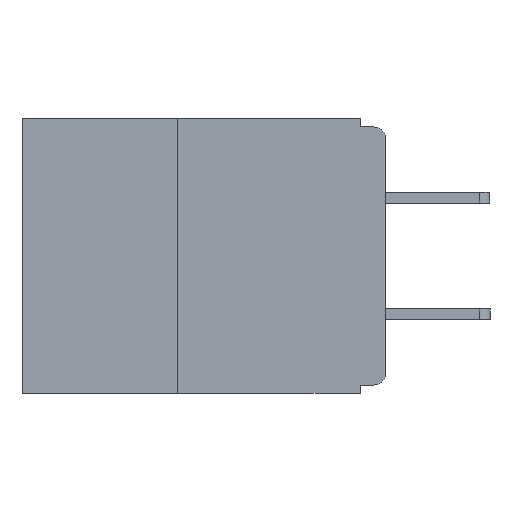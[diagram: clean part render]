
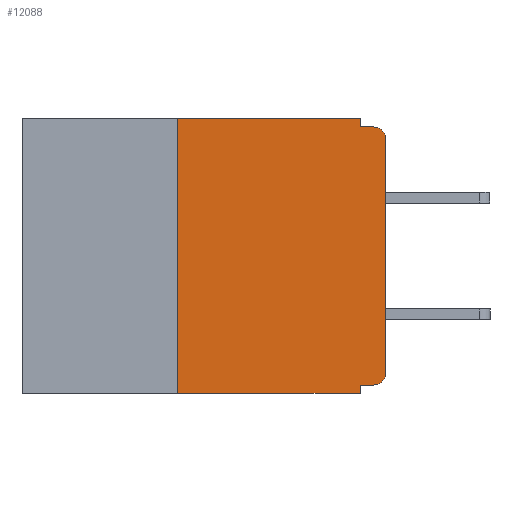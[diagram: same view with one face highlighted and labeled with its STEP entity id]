
A CAD part, left-side view. The second image highlights one B-rep face of the part: STEP entity #12088.
In plain terms, the highlighted planar face has unit normal (-1, 0, 0).
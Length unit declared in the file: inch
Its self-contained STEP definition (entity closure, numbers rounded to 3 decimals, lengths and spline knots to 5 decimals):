
#618 = VECTOR ( 'NONE', #12654, 39.37008 ) ;
#754 = DIRECTION ( 'NONE',  ( -1., 0., 0. ) ) ;
#861 = DIRECTION ( 'NONE',  ( 0., -1., 0. ) ) ;
#1012 = VECTOR ( 'NONE', #10283, 39.37008 ) ;
#1029 = EDGE_CURVE ( 'NONE', #26435, #22996, #21744, .T. ) ;
#1649 = ORIENTED_EDGE ( 'NONE', *, *, #1029, .T. ) ;
#1729 = LINE ( 'NONE', #7966, #1012 ) ;
#2002 = VECTOR ( 'NONE', #13486, 39.37008 ) ;
#2051 = EDGE_CURVE ( 'NONE', #28417, #3940, #6034, .T. ) ;
#2320 = LINE ( 'NONE', #24086, #21237 ) ;
#3777 = CARTESIAN_POINT ( 'NONE',  ( 0., 0.25, 0. ) ) ;
#3940 = VERTEX_POINT ( 'NONE', #28882 ) ;
#4041 = VECTOR ( 'NONE', #9494, 39.37008 ) ;
#5260 = EDGE_CURVE ( 'NONE', #5941, #18944, #28084, .T. ) ;
#5427 = ORIENTED_EDGE ( 'NONE', *, *, #2051, .F. ) ;
#5639 = VERTEX_POINT ( 'NONE', #13345 ) ;
#5941 = VERTEX_POINT ( 'NONE', #7486 ) ;
#6034 = LINE ( 'NONE', #12742, #618 ) ;
#6100 = ORIENTED_EDGE ( 'NONE', *, *, #17525, .F. ) ;
#6340 = ORIENTED_EDGE ( 'NONE', *, *, #19061, .T. ) ;
#6968 = VECTOR ( 'NONE', #24032, 39.37008 ) ;
#7220 = CIRCLE ( 'NONE', #20541, 0.015 ) ;
#7486 = CARTESIAN_POINT ( 'NONE',  ( 0., 0.031, -0.32 ) ) ;
#7966 = CARTESIAN_POINT ( 'NONE',  ( 0., 0.437, -0.33 ) ) ;
#8634 = CARTESIAN_POINT ( 'NONE',  ( 0., 0.031, -0.33 ) ) ;
#8992 = CARTESIAN_POINT ( 'NONE',  ( 0., 0.031, -0.33 ) ) ;
#9402 = ORIENTED_EDGE ( 'NONE', *, *, #26508, .F. ) ;
#9494 = DIRECTION ( 'NONE',  ( 0., 0., -1. ) ) ;
#9524 = PLANE ( 'NONE',  #17024 ) ;
#10270 = ORIENTED_EDGE ( 'NONE', *, *, #23504, .T. ) ;
#10283 = DIRECTION ( 'NONE',  ( 0., -1., 0. ) ) ;
#10932 = ORIENTED_EDGE ( 'NONE', *, *, #14489, .F. ) ;
#11185 = CARTESIAN_POINT ( 'NONE',  ( 0., 0.25, -0.33 ) ) ;
#11300 = ORIENTED_EDGE ( 'NONE', *, *, #15483, .F. ) ;
#11381 = DIRECTION ( 'NONE',  ( -1., 0., 0. ) ) ;
#11862 = DIRECTION ( 'NONE',  ( 0., 0., -1. ) ) ;
#12088 = ADVANCED_FACE ( 'NONE', ( #17539 ), #9524, .F. ) ;
#12172 = CIRCLE ( 'NONE', #22518, 0.015 ) ;
#12307 = CARTESIAN_POINT ( 'NONE',  ( 0., 0., -0.025 ) ) ;
#12654 = DIRECTION ( 'NONE',  ( 0., -1., 0. ) ) ;
#12742 = CARTESIAN_POINT ( 'NONE',  ( 0., 0.437, 0. ) ) ;
#12749 = VECTOR ( 'NONE', #861, 39.37008 ) ;
#12937 = EDGE_CURVE ( 'NONE', #25260, #18944, #1729, .T. ) ;
#13345 = CARTESIAN_POINT ( 'NONE',  ( 0., 0.031, -0.01 ) ) ;
#13359 = ORIENTED_EDGE ( 'NONE', *, *, #5260, .F. ) ;
#13463 = LINE ( 'NONE', #28009, #12749 ) ;
#13486 = DIRECTION ( 'NONE',  ( 0., 0., 1. ) ) ;
#14032 = VERTEX_POINT ( 'NONE', #18706 ) ;
#14081 = CARTESIAN_POINT ( 'NONE',  ( 0., 0.437, 0. ) ) ;
#14489 = EDGE_CURVE ( 'NONE', #25260, #28417, #26154, .T. ) ;
#14545 = CARTESIAN_POINT ( 'NONE',  ( 0., 0.015, -0.025 ) ) ;
#14838 = CARTESIAN_POINT ( 'NONE',  ( 0., 0., -0.305 ) ) ;
#14895 = DIRECTION ( 'NONE',  ( 0., 0., 1. ) ) ;
#15483 = EDGE_CURVE ( 'NONE', #5639, #14032, #13463, .T. ) ;
#15661 = VERTEX_POINT ( 'NONE', #28649 ) ;
#15788 = VECTOR ( 'NONE', #14895, 39.37008 ) ;
#16414 = EDGE_LOOP ( 'NONE', ( #1649, #10270, #11300, #6100, #5427, #10932, #20932, #13359, #9402, #6340 ) ) ;
#16831 = DIRECTION ( 'NONE',  ( 0., 0., -1. ) ) ;
#17024 = AXIS2_PLACEMENT_3D ( 'NONE', #14081, #25323, #11862 ) ;
#17499 = DIRECTION ( 'NONE',  ( 0., 1., 0. ) ) ;
#17525 = EDGE_CURVE ( 'NONE', #3940, #5639, #25732, .T. ) ;
#17539 = FACE_OUTER_BOUND ( 'NONE', #16414, .T. ) ;
#18324 = CARTESIAN_POINT ( 'NONE',  ( 0., 0., 0. ) ) ;
#18706 = CARTESIAN_POINT ( 'NONE',  ( 0., 0.015, -0.01 ) ) ;
#18944 = VERTEX_POINT ( 'NONE', #8634 ) ;
#19061 = EDGE_CURVE ( 'NONE', #15661, #26435, #7220, .T. ) ;
#20541 = AXIS2_PLACEMENT_3D ( 'NONE', #24844, #11381, #27095 ) ;
#20932 = ORIENTED_EDGE ( 'NONE', *, *, #12937, .T. ) ;
#21237 = VECTOR ( 'NONE', #17499, 39.37008 ) ;
#21744 = LINE ( 'NONE', #18324, #15788 ) ;
#21825 = CARTESIAN_POINT ( 'NONE',  ( 0., 0.031, 0. ) ) ;
#22518 = AXIS2_PLACEMENT_3D ( 'NONE', #14545, #754, #16831 ) ;
#22996 = VERTEX_POINT ( 'NONE', #12307 ) ;
#23504 = EDGE_CURVE ( 'NONE', #22996, #14032, #12172, .T. ) ;
#24032 = DIRECTION ( 'NONE',  ( 0., 0., -1. ) ) ;
#24086 = CARTESIAN_POINT ( 'NONE',  ( 0., 0., -0.32 ) ) ;
#24844 = CARTESIAN_POINT ( 'NONE',  ( 0., 0.015, -0.305 ) ) ;
#25260 = VERTEX_POINT ( 'NONE', #27922 ) ;
#25323 = DIRECTION ( 'NONE',  ( 1., 0., 0. ) ) ;
#25732 = LINE ( 'NONE', #21825, #6968 ) ;
#26154 = LINE ( 'NONE', #11185, #2002 ) ;
#26435 = VERTEX_POINT ( 'NONE', #14838 ) ;
#26508 = EDGE_CURVE ( 'NONE', #15661, #5941, #2320, .T. ) ;
#27095 = DIRECTION ( 'NONE',  ( 0., 0., -1. ) ) ;
#27922 = CARTESIAN_POINT ( 'NONE',  ( 0., 0.25, -0.33 ) ) ;
#28009 = CARTESIAN_POINT ( 'NONE',  ( 0., 0., -0.01 ) ) ;
#28084 = LINE ( 'NONE', #8992, #4041 ) ;
#28417 = VERTEX_POINT ( 'NONE', #3777 ) ;
#28649 = CARTESIAN_POINT ( 'NONE',  ( 0., 0.015, -0.32 ) ) ;
#28882 = CARTESIAN_POINT ( 'NONE',  ( 0., 0.031, 0. ) ) ;
